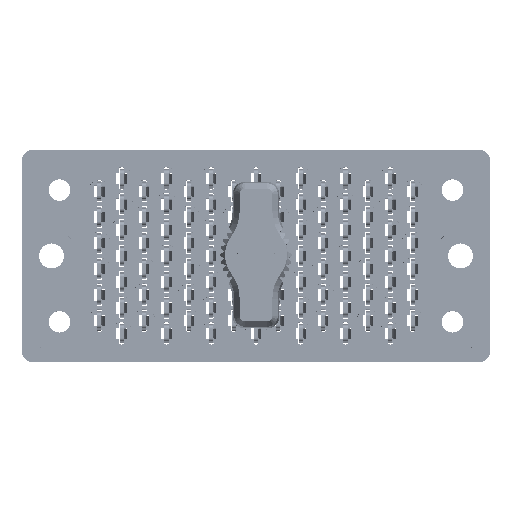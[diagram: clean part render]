
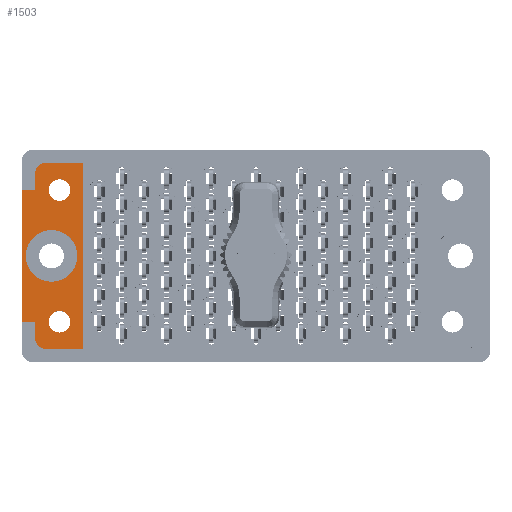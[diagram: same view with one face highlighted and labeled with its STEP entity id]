
A CAD part, top view. The second image highlights one B-rep face of the part: STEP entity #1503.
In plain terms, the highlighted planar face has unit normal (0, 0, 1).
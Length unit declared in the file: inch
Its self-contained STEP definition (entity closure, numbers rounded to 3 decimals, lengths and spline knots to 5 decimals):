
#1127 = CARTESIAN_POINT ( 'NONE',  ( -1.2825, 0.478, -0.117 ) ) ;
#1503 = ADVANCED_FACE ( 'NONE', ( #47606, #86518, #23363, #63367 ), #29447, .T. ) ;
#1650 = EDGE_CURVE ( 'NONE', #70452, #36390, #35949, .T. ) ;
#1840 = VERTEX_POINT ( 'NONE', #27030 ) ;
#2322 = CARTESIAN_POINT ( 'NONE',  ( 0., -0.54, -0.117 ) ) ;
#2570 = CARTESIAN_POINT ( 'NONE',  ( -1.2825, 0., -0.117 ) ) ;
#3572 = CARTESIAN_POINT ( 'NONE',  ( -1.005, 0.617, -0.117 ) ) ;
#3732 = DIRECTION ( 'NONE',  ( 1., 0., 0. ) ) ;
#4581 = CARTESIAN_POINT ( 'NONE',  ( -1.1875, 0., -0.117 ) ) ;
#4682 = EDGE_CURVE ( 'NONE', #36390, #17445, #68026, .T. ) ;
#6107 = CARTESIAN_POINT ( 'NONE',  ( -1.359, 0.617, -0.117 ) ) ;
#6698 = DIRECTION ( 'NONE',  ( -1., 0., 0. ) ) ;
#9386 = DIRECTION ( 'NONE',  ( -1., 0., 0. ) ) ;
#10359 = DIRECTION ( 'NONE',  ( 0., 1., 0. ) ) ;
#10774 = DIRECTION ( 'NONE',  ( -1., 0., 0. ) ) ;
#10942 = CARTESIAN_POINT ( 'NONE',  ( -1.141, 0.3825, -0.117 ) ) ;
#11044 = ORIENTED_EDGE ( 'NONE', *, *, #81124, .F. ) ;
#11592 = VERTEX_POINT ( 'NONE', #60611 ) ;
#12282 = DIRECTION ( 'NONE',  ( 1., 0., 0. ) ) ;
#12639 = ORIENTED_EDGE ( 'NONE', *, *, #46183, .T. ) ;
#12831 = VECTOR ( 'NONE', #84474, 39.37008 ) ;
#15143 = ORIENTED_EDGE ( 'NONE', *, *, #20067, .T. ) ;
#15358 = VECTOR ( 'NONE', #63763, 39.37008 ) ;
#15435 = VERTEX_POINT ( 'NONE', #26267 ) ;
#15723 = DIRECTION ( 'NONE',  ( 0., 0., 1. ) ) ;
#16225 = DIRECTION ( 'NONE',  ( 0., 0., 1. ) ) ;
#16699 = CARTESIAN_POINT ( 'NONE',  ( -1.2205, 0.478, -0.117 ) ) ;
#17445 = VERTEX_POINT ( 'NONE', #1127 ) ;
#17467 = VECTOR ( 'NONE', #10774, 39.37008 ) ;
#18011 = CARTESIAN_POINT ( 'NONE',  ( -1.005, -0.54, -0.117 ) ) ;
#18814 = DIRECTION ( 'NONE',  ( 0., -1., 0. ) ) ;
#19147 = EDGE_LOOP ( 'NONE', ( #71192, #87038, #47240, #12639, #31519, #35268, #81209, #31201, #15143, #11044 ) ) ;
#19372 = AXIS2_PLACEMENT_3D ( 'NONE', #16699, #63758, #31393 ) ;
#19584 = ORIENTED_EDGE ( 'NONE', *, *, #38364, .F. ) ;
#20067 = EDGE_CURVE ( 'NONE', #11592, #43227, #61277, .T. ) ;
#20297 = CARTESIAN_POINT ( 'NONE',  ( -1.141, -0.3825, -0.117 ) ) ;
#20642 = EDGE_CURVE ( 'NONE', #17445, #1840, #27521, .T. ) ;
#20753 = CIRCLE ( 'NONE', #66744, 0.062 ) ;
#21168 = CARTESIAN_POINT ( 'NONE',  ( -1.2035, -0.3825, -0.117 ) ) ;
#22431 = EDGE_CURVE ( 'NONE', #73483, #47639, #62054, .T. ) ;
#23363 = FACE_BOUND ( 'NONE', #24402, .T. ) ;
#24162 = AXIS2_PLACEMENT_3D ( 'NONE', #4581, #37885, #3732 ) ;
#24246 = CARTESIAN_POINT ( 'NONE',  ( -1.3375, 0., -0.117 ) ) ;
#24402 = EDGE_LOOP ( 'NONE', ( #19584, #80091 ) ) ;
#25728 = VECTOR ( 'NONE', #9386, 39.37008 ) ;
#26267 = CARTESIAN_POINT ( 'NONE',  ( -1.2035, 0.3825, -0.117 ) ) ;
#26382 = DIRECTION ( 'NONE',  ( 0., 0., 1. ) ) ;
#27030 = CARTESIAN_POINT ( 'NONE',  ( -1.2825, 0.3825, -0.117 ) ) ;
#27521 = LINE ( 'NONE', #66074, #61191 ) ;
#28589 = DIRECTION ( 'NONE',  ( 0., 0., 1. ) ) ;
#29447 = PLANE ( 'NONE',  #66493 ) ;
#30156 = DIRECTION ( 'NONE',  ( 0., 0., 1. ) ) ;
#30323 = VERTEX_POINT ( 'NONE', #49612 ) ;
#31025 = CARTESIAN_POINT ( 'NONE',  ( -1.141, -0.3825, -0.117 ) ) ;
#31062 = CARTESIAN_POINT ( 'NONE',  ( 0., -0.3825, -0.117 ) ) ;
#31201 = ORIENTED_EDGE ( 'NONE', *, *, #51069, .T. ) ;
#31393 = DIRECTION ( 'NONE',  ( 1., 0., 0. ) ) ;
#31519 = ORIENTED_EDGE ( 'NONE', *, *, #1650, .T. ) ;
#31765 = AXIS2_PLACEMENT_3D ( 'NONE', #83986, #43048, #49566 ) ;
#32562 = CARTESIAN_POINT ( 'NONE',  ( -1.141, 0.3825, -0.117 ) ) ;
#34669 = CIRCLE ( 'NONE', #55136, 0.0625 ) ;
#35268 = ORIENTED_EDGE ( 'NONE', *, *, #4682, .T. ) ;
#35290 = EDGE_CURVE ( 'NONE', #52987, #76779, #83216, .T. ) ;
#35949 = LINE ( 'NONE', #70898, #12831 ) ;
#36390 = VERTEX_POINT ( 'NONE', #50899 ) ;
#37265 = VERTEX_POINT ( 'NONE', #46324 ) ;
#37885 = DIRECTION ( 'NONE',  ( 0., 0., 1. ) ) ;
#38364 = EDGE_CURVE ( 'NONE', #47639, #73483, #39511, .T. ) ;
#38673 = CARTESIAN_POINT ( 'NONE',  ( -1.005, 0.54, -0.117 ) ) ;
#39511 = CIRCLE ( 'NONE', #24162, 0.15 ) ;
#40894 = AXIS2_PLACEMENT_3D ( 'NONE', #31025, #30156, #71039 ) ;
#40903 = CARTESIAN_POINT ( 'NONE',  ( -1.0785, -0.3825, -0.117 ) ) ;
#43048 = DIRECTION ( 'NONE',  ( 0., 0., 1. ) ) ;
#43227 = VERTEX_POINT ( 'NONE', #67872 ) ;
#46183 = EDGE_CURVE ( 'NONE', #48168, #70452, #79393, .T. ) ;
#46324 = CARTESIAN_POINT ( 'NONE',  ( -1.0785, 0.3825, -0.117 ) ) ;
#47240 = ORIENTED_EDGE ( 'NONE', *, *, #57279, .F. ) ;
#47350 = DIRECTION ( 'NONE',  ( 0., 0., 1. ) ) ;
#47606 = FACE_BOUND ( 'NONE', #74942, .T. ) ;
#47639 = VERTEX_POINT ( 'NONE', #86050 ) ;
#48063 = AXIS2_PLACEMENT_3D ( 'NONE', #20297, #47350, #53835 ) ;
#48168 = VERTEX_POINT ( 'NONE', #18011 ) ;
#48887 = DIRECTION ( 'NONE',  ( 1., 0., 0. ) ) ;
#48890 = DIRECTION ( 'NONE',  ( 1., 0., 0. ) ) ;
#49566 = DIRECTION ( 'NONE',  ( 1., 0., 0. ) ) ;
#49612 = CARTESIAN_POINT ( 'NONE',  ( -1.2825, -0.478, -0.117 ) ) ;
#50154 = ORIENTED_EDGE ( 'NONE', *, *, #35290, .F. ) ;
#50527 = CARTESIAN_POINT ( 'NONE',  ( -1.2205, -0.54, -0.117 ) ) ;
#50899 = CARTESIAN_POINT ( 'NONE',  ( -1.2205, 0.54, -0.117 ) ) ;
#51069 = EDGE_CURVE ( 'NONE', #1840, #11592, #64953, .T. ) ;
#52987 = VERTEX_POINT ( 'NONE', #40903 ) ;
#53064 = EDGE_LOOP ( 'NONE', ( #64267, #81629 ) ) ;
#53766 = VERTEX_POINT ( 'NONE', #50527 ) ;
#53835 = DIRECTION ( 'NONE',  ( 1., 0., 0. ) ) ;
#54771 = EDGE_CURVE ( 'NONE', #76779, #52987, #80012, .T. ) ;
#55136 = AXIS2_PLACEMENT_3D ( 'NONE', #10942, #16225, #48887 ) ;
#55709 = EDGE_CURVE ( 'NONE', #30323, #53766, #20753, .T. ) ;
#57279 = EDGE_CURVE ( 'NONE', #48168, #53766, #74080, .T. ) ;
#57659 = VECTOR ( 'NONE', #6698, 39.37008 ) ;
#60611 = CARTESIAN_POINT ( 'NONE',  ( -1.359, 0.3825, -0.117 ) ) ;
#61191 = VECTOR ( 'NONE', #72847, 39.37008 ) ;
#61277 = LINE ( 'NONE', #6107, #77059 ) ;
#61867 = CIRCLE ( 'NONE', #80771, 0.0625 ) ;
#62054 = CIRCLE ( 'NONE', #31765, 0.15 ) ;
#62775 = DIRECTION ( 'NONE',  ( 1., 0., 0. ) ) ;
#63367 = FACE_OUTER_BOUND ( 'NONE', #19147, .T. ) ;
#63758 = DIRECTION ( 'NONE',  ( 0., 0., 1. ) ) ;
#63763 = DIRECTION ( 'NONE',  ( 0., -1., 0. ) ) ;
#64267 = ORIENTED_EDGE ( 'NONE', *, *, #83430, .F. ) ;
#64953 = LINE ( 'NONE', #74086, #57659 ) ;
#66074 = CARTESIAN_POINT ( 'NONE',  ( -1.2825, 0., -0.117 ) ) ;
#66493 = AXIS2_PLACEMENT_3D ( 'NONE', #68887, #28589, #48890 ) ;
#66744 = AXIS2_PLACEMENT_3D ( 'NONE', #76027, #15723, #62775 ) ;
#67872 = CARTESIAN_POINT ( 'NONE',  ( -1.359, -0.3825, -0.117 ) ) ;
#68026 = CIRCLE ( 'NONE', #19372, 0.062 ) ;
#68887 = CARTESIAN_POINT ( 'NONE',  ( -1.359, -0.617, -0.117 ) ) ;
#69814 = VERTEX_POINT ( 'NONE', #78574 ) ;
#70452 = VERTEX_POINT ( 'NONE', #38673 ) ;
#70898 = CARTESIAN_POINT ( 'NONE',  ( 0., 0.54, -0.117 ) ) ;
#71039 = DIRECTION ( 'NONE',  ( 1., 0., 0. ) ) ;
#71192 = ORIENTED_EDGE ( 'NONE', *, *, #85505, .T. ) ;
#72392 = ORIENTED_EDGE ( 'NONE', *, *, #54771, .F. ) ;
#72847 = DIRECTION ( 'NONE',  ( 0., -1., 0. ) ) ;
#73483 = VERTEX_POINT ( 'NONE', #24246 ) ;
#74080 = LINE ( 'NONE', #2322, #25728 ) ;
#74086 = CARTESIAN_POINT ( 'NONE',  ( 0., 0.3825, -0.117 ) ) ;
#74942 = EDGE_LOOP ( 'NONE', ( #72392, #50154 ) ) ;
#76027 = CARTESIAN_POINT ( 'NONE',  ( -1.2205, -0.478, -0.117 ) ) ;
#76779 = VERTEX_POINT ( 'NONE', #21168 ) ;
#77059 = VECTOR ( 'NONE', #18814, 39.37008 ) ;
#78574 = CARTESIAN_POINT ( 'NONE',  ( -1.2825, -0.3825, -0.117 ) ) ;
#79393 = LINE ( 'NONE', #3572, #86727 ) ;
#80012 = CIRCLE ( 'NONE', #48063, 0.0625 ) ;
#80091 = ORIENTED_EDGE ( 'NONE', *, *, #22431, .F. ) ;
#80771 = AXIS2_PLACEMENT_3D ( 'NONE', #32562, #26382, #12282 ) ;
#81124 = EDGE_CURVE ( 'NONE', #69814, #43227, #84856, .T. ) ;
#81209 = ORIENTED_EDGE ( 'NONE', *, *, #20642, .T. ) ;
#81629 = ORIENTED_EDGE ( 'NONE', *, *, #84272, .F. ) ;
#82747 = LINE ( 'NONE', #2570, #15358 ) ;
#83216 = CIRCLE ( 'NONE', #40894, 0.0625 ) ;
#83430 = EDGE_CURVE ( 'NONE', #15435, #37265, #34669, .T. ) ;
#83986 = CARTESIAN_POINT ( 'NONE',  ( -1.1875, 0., -0.117 ) ) ;
#84272 = EDGE_CURVE ( 'NONE', #37265, #15435, #61867, .T. ) ;
#84474 = DIRECTION ( 'NONE',  ( -1., 0., 0. ) ) ;
#84856 = LINE ( 'NONE', #31062, #17467 ) ;
#85505 = EDGE_CURVE ( 'NONE', #69814, #30323, #82747, .T. ) ;
#86050 = CARTESIAN_POINT ( 'NONE',  ( -1.0375, 0., -0.117 ) ) ;
#86518 = FACE_BOUND ( 'NONE', #53064, .T. ) ;
#86727 = VECTOR ( 'NONE', #10359, 39.37008 ) ;
#87038 = ORIENTED_EDGE ( 'NONE', *, *, #55709, .T. ) ;
